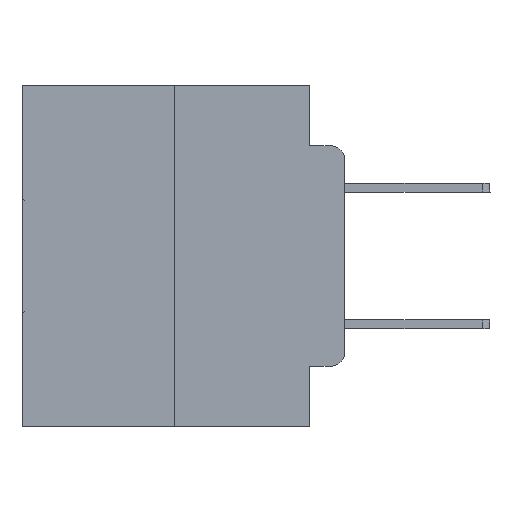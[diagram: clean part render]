
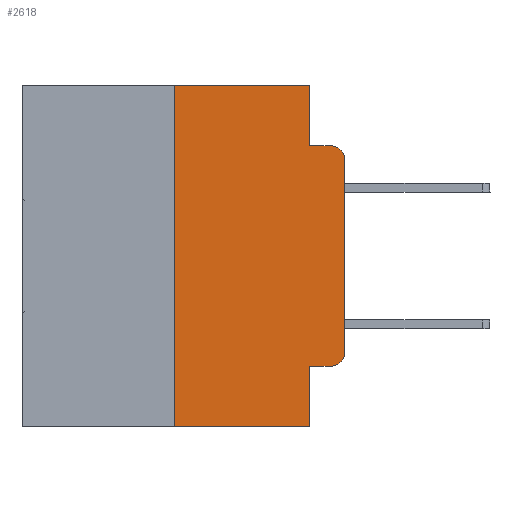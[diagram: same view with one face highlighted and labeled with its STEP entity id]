
A CAD part, left-side view. The second image highlights one B-rep face of the part: STEP entity #2618.
In plain terms, the highlighted planar face has unit normal (-1, 0, 0).
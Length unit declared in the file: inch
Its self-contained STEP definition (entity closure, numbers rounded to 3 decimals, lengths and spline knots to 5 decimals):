
#210 = VECTOR ( 'NONE', #8498, 39.37008 ) ;
#254 = VECTOR ( 'NONE', #16087, 39.37008 ) ;
#370 = CARTESIAN_POINT ( 'NONE',  ( 0., 0.051, -0.4115 ) ) ;
#706 = DIRECTION ( 'NONE',  ( 0., 0., -1. ) ) ;
#1066 = EDGE_CURVE ( 'NONE', #25162, #21007, #12036, .T. ) ;
#1310 = CARTESIAN_POINT ( 'NONE',  ( 0., 0.02, -0.3915 ) ) ;
#1825 = EDGE_CURVE ( 'NONE', #18151, #19563, #19131, .T. ) ;
#1865 = VECTOR ( 'NONE', #26899, 39.37008 ) ;
#2323 = LINE ( 'NONE', #28850, #18822 ) ;
#2559 = VERTEX_POINT ( 'NONE', #370 ) ;
#2618 = ADVANCED_FACE ( 'NONE', ( #5074 ), #21136, .F. ) ;
#3634 = DIRECTION ( 'NONE',  ( 0., 0., -1. ) ) ;
#4991 = CARTESIAN_POINT ( 'NONE',  ( 0., 0.051, 0. ) ) ;
#5074 = FACE_OUTER_BOUND ( 'NONE', #29460, .T. ) ;
#5908 = VECTOR ( 'NONE', #19630, 39.37008 ) ;
#5982 = CARTESIAN_POINT ( 'NONE',  ( 0., 0.473, -0.5 ) ) ;
#6359 = LINE ( 'NONE', #23151, #254 ) ;
#7376 = DIRECTION ( 'NONE',  ( 0., -1., 0. ) ) ;
#7867 = VERTEX_POINT ( 'NONE', #21263 ) ;
#8498 = DIRECTION ( 'NONE',  ( 0., 0., 1. ) ) ;
#8839 = ORIENTED_EDGE ( 'NONE', *, *, #17637, .T. ) ;
#10854 = CARTESIAN_POINT ( 'NONE',  ( 0., 0.051, -0.5 ) ) ;
#11325 = ORIENTED_EDGE ( 'NONE', *, *, #26629, .T. ) ;
#11553 = AXIS2_PLACEMENT_3D ( 'NONE', #1310, #26475, #3634 ) ;
#12036 = LINE ( 'NONE', #5982, #5908 ) ;
#12113 = EDGE_CURVE ( 'NONE', #2559, #21007, #23023, .T. ) ;
#12213 = ORIENTED_EDGE ( 'NONE', *, *, #15385, .F. ) ;
#13048 = VERTEX_POINT ( 'NONE', #24198 ) ;
#13295 = CARTESIAN_POINT ( 'NONE',  ( 0., 0.02, -0.0885 ) ) ;
#13380 = DIRECTION ( 'NONE',  ( 0., -1., 0. ) ) ;
#13482 = ORIENTED_EDGE ( 'NONE', *, *, #21827, .F. ) ;
#14409 = CARTESIAN_POINT ( 'NONE',  ( 0., 0.051, -0.0885 ) ) ;
#15330 = LINE ( 'NONE', #22292, #24274 ) ;
#15385 = EDGE_CURVE ( 'NONE', #19563, #27930, #6359, .T. ) ;
#15564 = VECTOR ( 'NONE', #7376, 39.37008 ) ;
#16087 = DIRECTION ( 'NONE',  ( 0., 0., -1. ) ) ;
#16331 = VERTEX_POINT ( 'NONE', #13295 ) ;
#16374 = LINE ( 'NONE', #27142, #210 ) ;
#16445 = ORIENTED_EDGE ( 'NONE', *, *, #1825, .F. ) ;
#16550 = DIRECTION ( 'NONE',  ( 0., 0., -1. ) ) ;
#16643 = ORIENTED_EDGE ( 'NONE', *, *, #29090, .T. ) ;
#16672 = CIRCLE ( 'NONE', #17933, 0.02 ) ;
#16740 = DIRECTION ( 'NONE',  ( -1., 0., 0. ) ) ;
#17047 = DIRECTION ( 'NONE',  ( 1., 0., 0. ) ) ;
#17637 = EDGE_CURVE ( 'NONE', #23517, #7867, #2323, .T. ) ;
#17690 = CIRCLE ( 'NONE', #11553, 0.02 ) ;
#17695 = VECTOR ( 'NONE', #18532, 39.37008 ) ;
#17933 = AXIS2_PLACEMENT_3D ( 'NONE', #25617, #16740, #16550 ) ;
#18017 = EDGE_CURVE ( 'NONE', #7867, #16331, #16672, .T. ) ;
#18151 = VERTEX_POINT ( 'NONE', #26235 ) ;
#18274 = ORIENTED_EDGE ( 'NONE', *, *, #1066, .T. ) ;
#18532 = DIRECTION ( 'NONE',  ( 0., -1., 0. ) ) ;
#18822 = VECTOR ( 'NONE', #19545, 39.37008 ) ;
#18981 = ORIENTED_EDGE ( 'NONE', *, *, #18017, .T. ) ;
#19131 = LINE ( 'NONE', #22615, #17695 ) ;
#19545 = DIRECTION ( 'NONE',  ( 0., 0., 1. ) ) ;
#19563 = VERTEX_POINT ( 'NONE', #4991 ) ;
#19630 = DIRECTION ( 'NONE',  ( 0., -1., 0. ) ) ;
#19682 = AXIS2_PLACEMENT_3D ( 'NONE', #28155, #17047, #706 ) ;
#19786 = CARTESIAN_POINT ( 'NONE',  ( 0., 0.25, -0.5 ) ) ;
#21007 = VERTEX_POINT ( 'NONE', #10854 ) ;
#21136 = PLANE ( 'NONE',  #19682 ) ;
#21263 = CARTESIAN_POINT ( 'NONE',  ( 0., 0., -0.1085 ) ) ;
#21827 = EDGE_CURVE ( 'NONE', #27930, #16331, #29152, .T. ) ;
#22245 = CARTESIAN_POINT ( 'NONE',  ( 0., 0.051, 0. ) ) ;
#22292 = CARTESIAN_POINT ( 'NONE',  ( 0., 0.051, -0.4115 ) ) ;
#22615 = CARTESIAN_POINT ( 'NONE',  ( 0., 0.473, 0. ) ) ;
#23023 = LINE ( 'NONE', #22245, #1865 ) ;
#23151 = CARTESIAN_POINT ( 'NONE',  ( 0., 0.051, 0. ) ) ;
#23517 = VERTEX_POINT ( 'NONE', #27022 ) ;
#24198 = CARTESIAN_POINT ( 'NONE',  ( 0., 0.02, -0.4115 ) ) ;
#24274 = VECTOR ( 'NONE', #13380, 39.37008 ) ;
#25162 = VERTEX_POINT ( 'NONE', #19786 ) ;
#25617 = CARTESIAN_POINT ( 'NONE',  ( 0., 0.02, -0.1085 ) ) ;
#25905 = EDGE_CURVE ( 'NONE', #25162, #18151, #16374, .T. ) ;
#26235 = CARTESIAN_POINT ( 'NONE',  ( 0., 0.25, 0. ) ) ;
#26398 = ORIENTED_EDGE ( 'NONE', *, *, #25905, .F. ) ;
#26475 = DIRECTION ( 'NONE',  ( -1., 0., 0. ) ) ;
#26629 = EDGE_CURVE ( 'NONE', #2559, #13048, #15330, .T. ) ;
#26899 = DIRECTION ( 'NONE',  ( 0., 0., -1. ) ) ;
#27022 = CARTESIAN_POINT ( 'NONE',  ( 0., 0., -0.3915 ) ) ;
#27142 = CARTESIAN_POINT ( 'NONE',  ( 0., 0.25, 0. ) ) ;
#27632 = ORIENTED_EDGE ( 'NONE', *, *, #12113, .F. ) ;
#27930 = VERTEX_POINT ( 'NONE', #28440 ) ;
#28155 = CARTESIAN_POINT ( 'NONE',  ( 0., 0.473, 0. ) ) ;
#28440 = CARTESIAN_POINT ( 'NONE',  ( 0., 0.051, -0.0885 ) ) ;
#28850 = CARTESIAN_POINT ( 'NONE',  ( 0., 0., 0. ) ) ;
#29090 = EDGE_CURVE ( 'NONE', #13048, #23517, #17690, .T. ) ;
#29152 = LINE ( 'NONE', #14409, #15564 ) ;
#29460 = EDGE_LOOP ( 'NONE', ( #8839, #18981, #13482, #12213, #16445, #26398, #18274, #27632, #11325, #16643 ) ) ;
